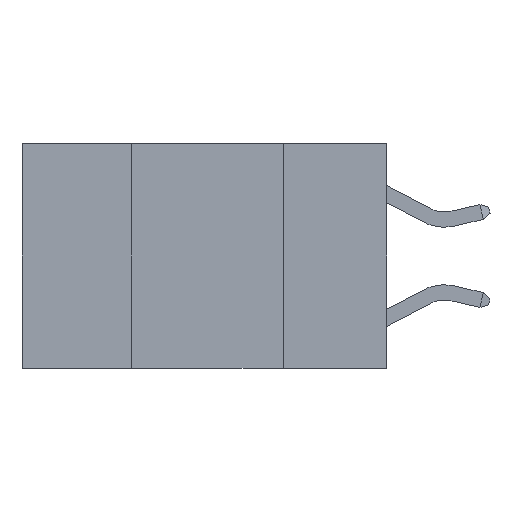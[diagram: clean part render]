
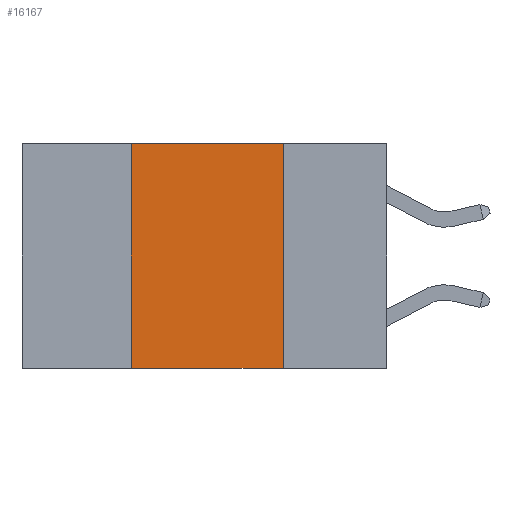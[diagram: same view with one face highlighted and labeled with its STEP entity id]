
A CAD part, left-side view. The second image highlights one B-rep face of the part: STEP entity #16167.
In plain terms, the highlighted planar face has unit normal (-1, 0, 0).
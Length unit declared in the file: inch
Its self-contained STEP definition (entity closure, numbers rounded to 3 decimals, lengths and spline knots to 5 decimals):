
#582 = CARTESIAN_POINT ( 'NONE',  ( 0., 0.42, 0. ) ) ;
#1414 = ORIENTED_EDGE ( 'NONE', *, *, #31473, .F. ) ;
#1692 = CARTESIAN_POINT ( 'NONE',  ( 0., 0.6, -0.37 ) ) ;
#2787 = VECTOR ( 'NONE', #26220, 39.37008 ) ;
#2891 = PLANE ( 'NONE',  #18633 ) ;
#3076 = VECTOR ( 'NONE', #28803, 39.37008 ) ;
#6302 = VERTEX_POINT ( 'NONE', #582 ) ;
#7246 = ORIENTED_EDGE ( 'NONE', *, *, #24893, .F. ) ;
#7841 = CARTESIAN_POINT ( 'NONE',  ( 0., 0.42, -0.37 ) ) ;
#7869 = CARTESIAN_POINT ( 'NONE',  ( 0., 0.6, 0. ) ) ;
#9173 = CARTESIAN_POINT ( 'NONE',  ( 0., 0.42, 0. ) ) ;
#10265 = VECTOR ( 'NONE', #23791, 39.37008 ) ;
#10306 = DIRECTION ( 'NONE',  ( 0., 0., -1. ) ) ;
#10358 = DIRECTION ( 'NONE',  ( 0., 0., -1. ) ) ;
#11046 = LINE ( 'NONE', #31097, #10265 ) ;
#11880 = VERTEX_POINT ( 'NONE', #26073 ) ;
#12539 = LINE ( 'NONE', #17628, #24858 ) ;
#16167 = ADVANCED_FACE ( 'NONE', ( #27258 ), #2891, .F. ) ;
#16228 = LINE ( 'NONE', #9173, #3076 ) ;
#16794 = VERTEX_POINT ( 'NONE', #7841 ) ;
#17032 = CARTESIAN_POINT ( 'NONE',  ( 0., 0.17, 0. ) ) ;
#17628 = CARTESIAN_POINT ( 'NONE',  ( 0., 0.17, 0. ) ) ;
#18633 = AXIS2_PLACEMENT_3D ( 'NONE', #7869, #25127, #10358 ) ;
#20337 = ORIENTED_EDGE ( 'NONE', *, *, #20583, .F. ) ;
#20583 = EDGE_CURVE ( 'NONE', #6302, #26031, #11046, .T. ) ;
#23249 = EDGE_CURVE ( 'NONE', #16794, #11880, #27506, .T. ) ;
#23791 = DIRECTION ( 'NONE',  ( 0., -1., 0. ) ) ;
#24858 = VECTOR ( 'NONE', #10306, 39.37008 ) ;
#24893 = EDGE_CURVE ( 'NONE', #26031, #11880, #12539, .T. ) ;
#25127 = DIRECTION ( 'NONE',  ( 1., 0., 0. ) ) ;
#26031 = VERTEX_POINT ( 'NONE', #17032 ) ;
#26073 = CARTESIAN_POINT ( 'NONE',  ( 0., 0.17, -0.37 ) ) ;
#26220 = DIRECTION ( 'NONE',  ( 0., -1., 0. ) ) ;
#27258 = FACE_OUTER_BOUND ( 'NONE', #28087, .T. ) ;
#27506 = LINE ( 'NONE', #1692, #2787 ) ;
#28087 = EDGE_LOOP ( 'NONE', ( #7246, #20337, #1414, #28484 ) ) ;
#28484 = ORIENTED_EDGE ( 'NONE', *, *, #23249, .T. ) ;
#28803 = DIRECTION ( 'NONE',  ( 0., 0., 1. ) ) ;
#31097 = CARTESIAN_POINT ( 'NONE',  ( 0., 0.6, 0. ) ) ;
#31473 = EDGE_CURVE ( 'NONE', #16794, #6302, #16228, .T. ) ;
